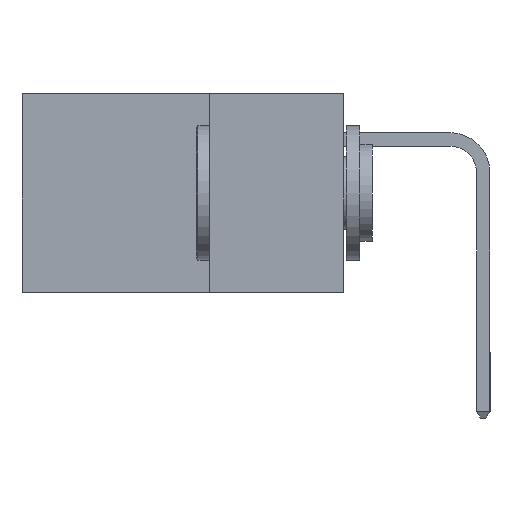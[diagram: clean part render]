
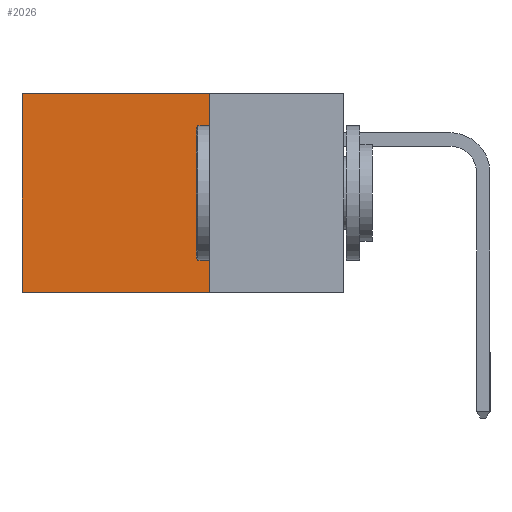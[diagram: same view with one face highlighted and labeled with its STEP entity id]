
A CAD part, left-side view. The second image highlights one B-rep face of the part: STEP entity #2026.
In plain terms, the highlighted planar face has unit normal (-1, 0, 0).
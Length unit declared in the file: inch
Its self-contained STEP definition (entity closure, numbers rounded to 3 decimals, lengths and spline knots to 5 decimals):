
#690 = DIRECTION ( 'NONE',  ( 0., 1., 0. ) ) ;
#970 = EDGE_LOOP ( 'NONE', ( #5241, #9739, #2267, #3250 ) ) ;
#1085 = CARTESIAN_POINT ( 'NONE',  ( 0.2615, 0.6, -0.37 ) ) ;
#1210 = VECTOR ( 'NONE', #690, 39.37008 ) ;
#2026 = ADVANCED_FACE ( 'NONE', ( #15642 ), #7614, .F. ) ;
#2267 = ORIENTED_EDGE ( 'NONE', *, *, #6910, .F. ) ;
#2270 = DIRECTION ( 'NONE',  ( 1., 0., 0. ) ) ;
#2441 = EDGE_CURVE ( 'NONE', #16462, #10541, #9788, .T. ) ;
#2743 = CARTESIAN_POINT ( 'NONE',  ( 0.2615, 0.6, 0. ) ) ;
#2745 = DIRECTION ( 'NONE',  ( 0., 0., -1. ) ) ;
#3004 = VECTOR ( 'NONE', #6331, 39.37008 ) ;
#3171 = AXIS2_PLACEMENT_3D ( 'NONE', #15560, #2270, #12915 ) ;
#3239 = VECTOR ( 'NONE', #7592, 39.37008 ) ;
#3250 = ORIENTED_EDGE ( 'NONE', *, *, #16527, .T. ) ;
#3577 = CARTESIAN_POINT ( 'NONE',  ( 0.2615, 0.25, -0.37 ) ) ;
#3580 = CARTESIAN_POINT ( 'NONE',  ( 0.2615, 0.6, -0.37 ) ) ;
#4553 = VERTEX_POINT ( 'NONE', #2743 ) ;
#4925 = LINE ( 'NONE', #12946, #3004 ) ;
#5241 = ORIENTED_EDGE ( 'NONE', *, *, #8112, .T. ) ;
#5943 = LINE ( 'NONE', #3577, #3239 ) ;
#6331 = DIRECTION ( 'NONE',  ( 0., 1., 0. ) ) ;
#6420 = CARTESIAN_POINT ( 'NONE',  ( 0.2615, 0.25, -0.37 ) ) ;
#6910 = EDGE_CURVE ( 'NONE', #10485, #16462, #5943, .T. ) ;
#7592 = DIRECTION ( 'NONE',  ( 0., 0., -1. ) ) ;
#7614 = PLANE ( 'NONE',  #3171 ) ;
#8112 = EDGE_CURVE ( 'NONE', #4553, #10541, #13045, .T. ) ;
#9407 = VECTOR ( 'NONE', #2745, 39.37008 ) ;
#9739 = ORIENTED_EDGE ( 'NONE', *, *, #2441, .F. ) ;
#9788 = LINE ( 'NONE', #15097, #1210 ) ;
#10485 = VERTEX_POINT ( 'NONE', #11422 ) ;
#10541 = VERTEX_POINT ( 'NONE', #3580 ) ;
#11422 = CARTESIAN_POINT ( 'NONE',  ( 0.2615, 0.25, 0. ) ) ;
#12915 = DIRECTION ( 'NONE',  ( 0., 0., -1. ) ) ;
#12946 = CARTESIAN_POINT ( 'NONE',  ( 0.2615, 0.25, 0. ) ) ;
#13045 = LINE ( 'NONE', #1085, #9407 ) ;
#15097 = CARTESIAN_POINT ( 'NONE',  ( 0.2615, 0.25, -0.37 ) ) ;
#15560 = CARTESIAN_POINT ( 'NONE',  ( 0.2615, 0.25, -0.37 ) ) ;
#15642 = FACE_OUTER_BOUND ( 'NONE', #970, .T. ) ;
#16462 = VERTEX_POINT ( 'NONE', #6420 ) ;
#16527 = EDGE_CURVE ( 'NONE', #10485, #4553, #4925, .T. ) ;
